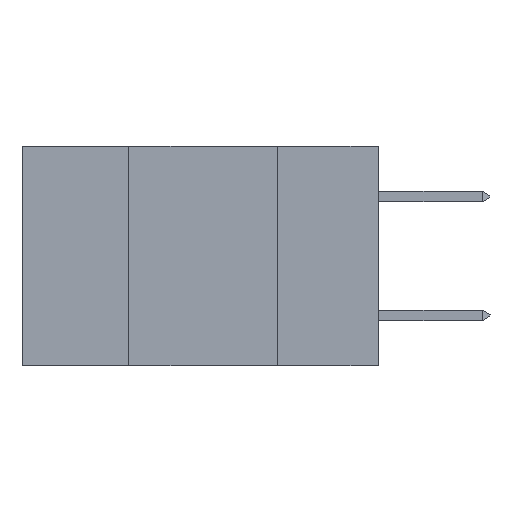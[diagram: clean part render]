
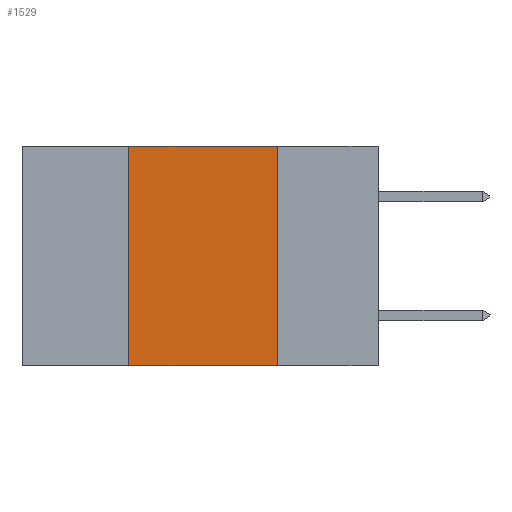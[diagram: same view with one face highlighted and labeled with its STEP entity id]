
A CAD part, left-side view. The second image highlights one B-rep face of the part: STEP entity #1529.
In plain terms, the highlighted planar face has unit normal (-1, 0, 0).
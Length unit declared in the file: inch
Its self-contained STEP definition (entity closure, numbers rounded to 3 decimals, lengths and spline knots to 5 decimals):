
#18 = VECTOR ( 'NONE', #7469, 39.37008 ) ;
#711 = EDGE_CURVE ( 'NONE', #8059, #1458, #9463, .T. ) ;
#1458 = VERTEX_POINT ( 'NONE', #11326 ) ;
#1529 = ADVANCED_FACE ( 'NONE', ( #4960 ), #10302, .F. ) ;
#2066 = EDGE_CURVE ( 'NONE', #6983, #6061, #7855, .T. ) ;
#2167 = ORIENTED_EDGE ( 'NONE', *, *, #711, .F. ) ;
#2391 = DIRECTION ( 'NONE',  ( 0., 0., -1. ) ) ;
#2763 = VECTOR ( 'NONE', #10236, 39.37008 ) ;
#4882 = AXIS2_PLACEMENT_3D ( 'NONE', #11149, #8248, #2391 ) ;
#4960 = FACE_OUTER_BOUND ( 'NONE', #10950, .T. ) ;
#5251 = ORIENTED_EDGE ( 'NONE', *, *, #2066, .F. ) ;
#5580 = VECTOR ( 'NONE', #9653, 39.37008 ) ;
#5652 = CARTESIAN_POINT ( 'NONE',  ( 0., 0.17, -0.37 ) ) ;
#5842 = EDGE_CURVE ( 'NONE', #8059, #6061, #9488, .T. ) ;
#6061 = VERTEX_POINT ( 'NONE', #5652 ) ;
#6212 = ORIENTED_EDGE ( 'NONE', *, *, #9249, .F. ) ;
#6741 = CARTESIAN_POINT ( 'NONE',  ( 0., 0.6, -0.37 ) ) ;
#6911 = DIRECTION ( 'NONE',  ( 0., -1., 0. ) ) ;
#6983 = VERTEX_POINT ( 'NONE', #10276 ) ;
#7469 = DIRECTION ( 'NONE',  ( 0., 0., -1. ) ) ;
#7600 = ORIENTED_EDGE ( 'NONE', *, *, #5842, .T. ) ;
#7855 = LINE ( 'NONE', #11315, #18 ) ;
#8009 = CARTESIAN_POINT ( 'NONE',  ( 0., 0.42, -0.37 ) ) ;
#8059 = VERTEX_POINT ( 'NONE', #8009 ) ;
#8248 = DIRECTION ( 'NONE',  ( 1., 0., 0. ) ) ;
#8541 = VECTOR ( 'NONE', #6911, 39.37008 ) ;
#9249 = EDGE_CURVE ( 'NONE', #1458, #6983, #11893, .T. ) ;
#9276 = CARTESIAN_POINT ( 'NONE',  ( 0., 0.6, 0. ) ) ;
#9463 = LINE ( 'NONE', #10563, #5580 ) ;
#9488 = LINE ( 'NONE', #6741, #8541 ) ;
#9653 = DIRECTION ( 'NONE',  ( 0., 0., 1. ) ) ;
#10236 = DIRECTION ( 'NONE',  ( 0., -1., 0. ) ) ;
#10276 = CARTESIAN_POINT ( 'NONE',  ( 0., 0.17, 0. ) ) ;
#10302 = PLANE ( 'NONE',  #4882 ) ;
#10563 = CARTESIAN_POINT ( 'NONE',  ( 0., 0.42, 0. ) ) ;
#10950 = EDGE_LOOP ( 'NONE', ( #5251, #6212, #2167, #7600 ) ) ;
#11149 = CARTESIAN_POINT ( 'NONE',  ( 0., 0.6, 0. ) ) ;
#11315 = CARTESIAN_POINT ( 'NONE',  ( 0., 0.17, 0. ) ) ;
#11326 = CARTESIAN_POINT ( 'NONE',  ( 0., 0.42, 0. ) ) ;
#11893 = LINE ( 'NONE', #9276, #2763 ) ;
